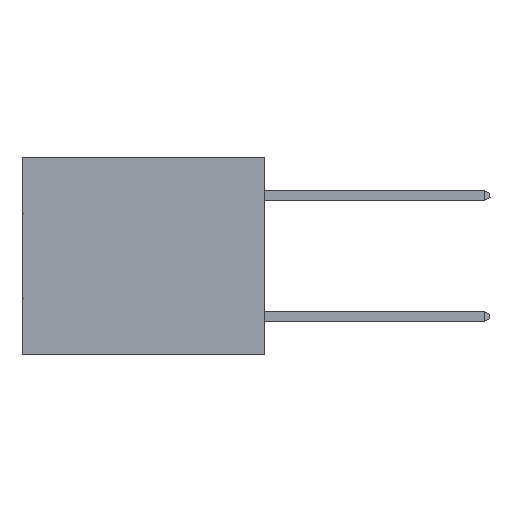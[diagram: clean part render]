
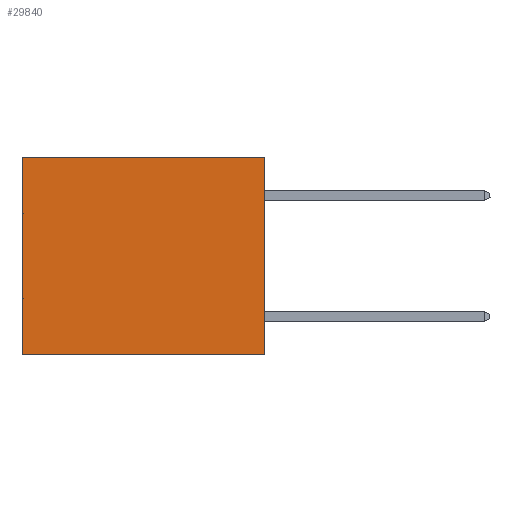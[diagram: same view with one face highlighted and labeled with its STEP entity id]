
A CAD part, left-side view. The second image highlights one B-rep face of the part: STEP entity #29840.
In plain terms, the highlighted planar face has unit normal (-1, 0, 0).
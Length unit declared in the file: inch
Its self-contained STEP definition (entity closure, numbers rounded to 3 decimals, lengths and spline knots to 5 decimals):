
#249 = VECTOR ( 'NONE', #22923, 39.37008 ) ;
#350 = VECTOR ( 'NONE', #3544, 39.37008 ) ;
#2363 = CARTESIAN_POINT ( 'NONE',  ( 0.3165, 0., -0.49 ) ) ;
#2936 = ORIENTED_EDGE ( 'NONE', *, *, #30752, .T. ) ;
#3010 = VERTEX_POINT ( 'NONE', #35416 ) ;
#3544 = DIRECTION ( 'NONE',  ( 0., 1., 0. ) ) ;
#4388 = PLANE ( 'NONE',  #33877 ) ;
#4624 = DIRECTION ( 'NONE',  ( 1., 0., 0. ) ) ;
#6034 = LINE ( 'NONE', #6384, #350 ) ;
#6384 = CARTESIAN_POINT ( 'NONE',  ( 0.3165, 0., 0. ) ) ;
#6430 = LINE ( 'NONE', #2363, #249 ) ;
#8205 = LINE ( 'NONE', #28062, #33846 ) ;
#8290 = ORIENTED_EDGE ( 'NONE', *, *, #29605, .F. ) ;
#9633 = ORIENTED_EDGE ( 'NONE', *, *, #24074, .F. ) ;
#9852 = EDGE_CURVE ( 'NONE', #3010, #23183, #8205, .T. ) ;
#9869 = CARTESIAN_POINT ( 'NONE',  ( 0.3165, 0.6, -0.49 ) ) ;
#11037 = CARTESIAN_POINT ( 'NONE',  ( 0.3165, 0., -0.49 ) ) ;
#14519 = LINE ( 'NONE', #11037, #18099 ) ;
#15461 = CARTESIAN_POINT ( 'NONE',  ( 0.3165, 0., -0.49 ) ) ;
#17091 = VERTEX_POINT ( 'NONE', #21005 ) ;
#17187 = DIRECTION ( 'NONE',  ( 0., 0., -1. ) ) ;
#18099 = VECTOR ( 'NONE', #30816, 39.37008 ) ;
#21005 = CARTESIAN_POINT ( 'NONE',  ( 0.3165, 0., 0. ) ) ;
#22164 = CARTESIAN_POINT ( 'NONE',  ( 0.3165, 0., -0.49 ) ) ;
#22476 = FACE_OUTER_BOUND ( 'NONE', #35476, .T. ) ;
#22923 = DIRECTION ( 'NONE',  ( 0., 0., -1. ) ) ;
#23183 = VERTEX_POINT ( 'NONE', #9869 ) ;
#24074 = EDGE_CURVE ( 'NONE', #17091, #27329, #6430, .T. ) ;
#27321 = ORIENTED_EDGE ( 'NONE', *, *, #9852, .T. ) ;
#27329 = VERTEX_POINT ( 'NONE', #22164 ) ;
#28062 = CARTESIAN_POINT ( 'NONE',  ( 0.3165, 0.6, -0.49 ) ) ;
#29605 = EDGE_CURVE ( 'NONE', #27329, #23183, #14519, .T. ) ;
#29840 = ADVANCED_FACE ( 'NONE', ( #22476 ), #4388, .F. ) ;
#30752 = EDGE_CURVE ( 'NONE', #17091, #3010, #6034, .T. ) ;
#30816 = DIRECTION ( 'NONE',  ( 0., 1., 0. ) ) ;
#33846 = VECTOR ( 'NONE', #17187, 39.37008 ) ;
#33877 = AXIS2_PLACEMENT_3D ( 'NONE', #15461, #4624, #35278 ) ;
#35278 = DIRECTION ( 'NONE',  ( 0., 0., -1. ) ) ;
#35416 = CARTESIAN_POINT ( 'NONE',  ( 0.3165, 0.6, 0. ) ) ;
#35476 = EDGE_LOOP ( 'NONE', ( #27321, #8290, #9633, #2936 ) ) ;
